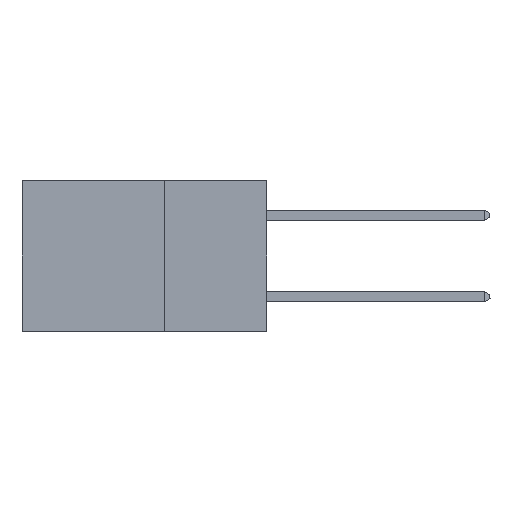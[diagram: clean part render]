
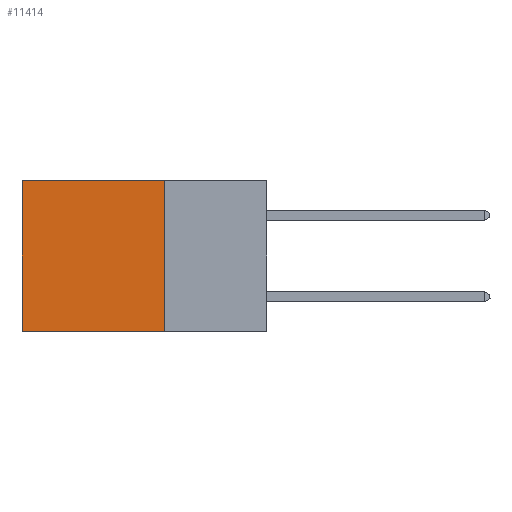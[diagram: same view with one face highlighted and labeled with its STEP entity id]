
A CAD part, left-side view. The second image highlights one B-rep face of the part: STEP entity #11414.
In plain terms, the highlighted planar face has unit normal (-1, 0, 0).
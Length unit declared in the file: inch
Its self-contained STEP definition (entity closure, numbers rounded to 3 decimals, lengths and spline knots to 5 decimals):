
#480 = CARTESIAN_POINT ( 'NONE',  ( 0.2875, 0.25, 0. ) ) ;
#610 = EDGE_CURVE ( 'NONE', #13612, #13038, #5426, .T. ) ;
#1691 = CARTESIAN_POINT ( 'NONE',  ( 0.2875, 0.25, 0. ) ) ;
#1906 = VECTOR ( 'NONE', #16756, 39.37008 ) ;
#2182 = ORIENTED_EDGE ( 'NONE', *, *, #17755, .F. ) ;
#2488 = CARTESIAN_POINT ( 'NONE',  ( 0.2875, 0.25, -0.37 ) ) ;
#3095 = FACE_OUTER_BOUND ( 'NONE', #14546, .T. ) ;
#4431 = VECTOR ( 'NONE', #12383, 39.37008 ) ;
#5426 = LINE ( 'NONE', #1691, #18476 ) ;
#5465 = CARTESIAN_POINT ( 'NONE',  ( 0.2875, 0.6, 0. ) ) ;
#6375 = ORIENTED_EDGE ( 'NONE', *, *, #6678, .T. ) ;
#6425 = LINE ( 'NONE', #11646, #1906 ) ;
#6678 = EDGE_CURVE ( 'NONE', #13038, #18874, #18069, .T. ) ;
#8005 = CARTESIAN_POINT ( 'NONE',  ( 0.2875, 0.25, 0. ) ) ;
#8462 = VECTOR ( 'NONE', #10160, 39.37008 ) ;
#9125 = EDGE_CURVE ( 'NONE', #13612, #14983, #17453, .T. ) ;
#9740 = DIRECTION ( 'NONE',  ( 1., 0., 0. ) ) ;
#10160 = DIRECTION ( 'NONE',  ( 0., 0., -1. ) ) ;
#10241 = ORIENTED_EDGE ( 'NONE', *, *, #610, .T. ) ;
#11414 = ADVANCED_FACE ( 'NONE', ( #3095 ), #18224, .F. ) ;
#11646 = CARTESIAN_POINT ( 'NONE',  ( 0.2875, 0.25, -0.37 ) ) ;
#12213 = ORIENTED_EDGE ( 'NONE', *, *, #9125, .F. ) ;
#12383 = DIRECTION ( 'NONE',  ( 0., 0., -1. ) ) ;
#13038 = VERTEX_POINT ( 'NONE', #17206 ) ;
#13612 = VERTEX_POINT ( 'NONE', #18542 ) ;
#14546 = EDGE_LOOP ( 'NONE', ( #6375, #2182, #12213, #10241 ) ) ;
#14955 = DIRECTION ( 'NONE',  ( 0., 1., 0. ) ) ;
#14983 = VERTEX_POINT ( 'NONE', #2488 ) ;
#15330 = AXIS2_PLACEMENT_3D ( 'NONE', #8005, #9740, #21559 ) ;
#16340 = CARTESIAN_POINT ( 'NONE',  ( 0.2875, 0.6, -0.37 ) ) ;
#16756 = DIRECTION ( 'NONE',  ( 0., 1., 0. ) ) ;
#17206 = CARTESIAN_POINT ( 'NONE',  ( 0.2875, 0.6, 0. ) ) ;
#17453 = LINE ( 'NONE', #480, #4431 ) ;
#17755 = EDGE_CURVE ( 'NONE', #14983, #18874, #6425, .T. ) ;
#18069 = LINE ( 'NONE', #5465, #8462 ) ;
#18224 = PLANE ( 'NONE',  #15330 ) ;
#18476 = VECTOR ( 'NONE', #14955, 39.37008 ) ;
#18542 = CARTESIAN_POINT ( 'NONE',  ( 0.2875, 0.25, 0. ) ) ;
#18874 = VERTEX_POINT ( 'NONE', #16340 ) ;
#21559 = DIRECTION ( 'NONE',  ( 0., 0., -1. ) ) ;
